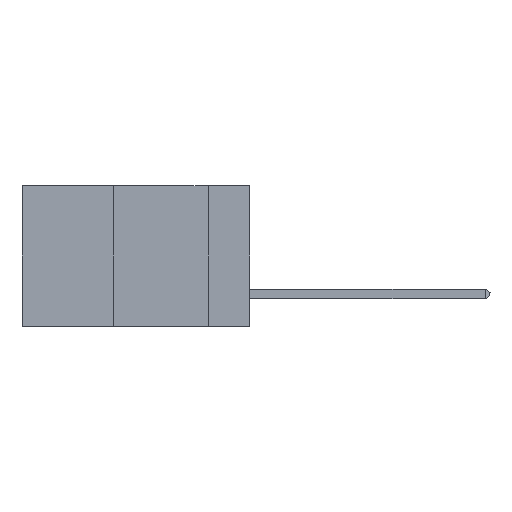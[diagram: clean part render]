
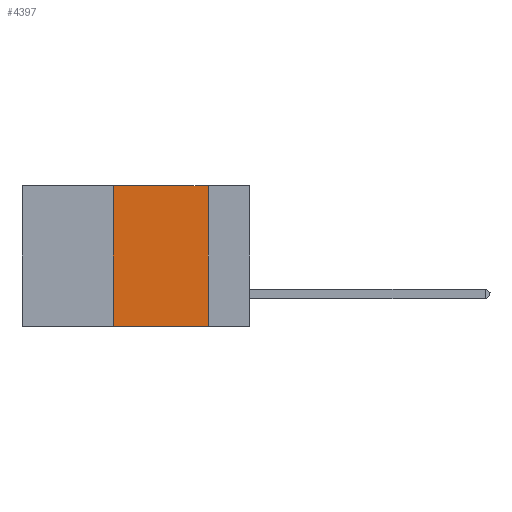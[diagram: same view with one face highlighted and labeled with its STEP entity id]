
A CAD part, left-side view. The second image highlights one B-rep face of the part: STEP entity #4397.
In plain terms, the highlighted planar face has unit normal (-1, 0, 0).
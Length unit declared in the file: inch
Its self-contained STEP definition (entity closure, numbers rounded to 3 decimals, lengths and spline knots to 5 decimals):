
#483 = DIRECTION ( 'NONE',  ( 0., -1., 0. ) ) ;
#1816 = FACE_OUTER_BOUND ( 'NONE', #12351, .T. ) ;
#2091 = ORIENTED_EDGE ( 'NONE', *, *, #14370, .T. ) ;
#2584 = DIRECTION ( 'NONE',  ( 0., 0., 1. ) ) ;
#3149 = DIRECTION ( 'NONE',  ( 0., 0., -1. ) ) ;
#3611 = CARTESIAN_POINT ( 'NONE',  ( 0., 0.36, -0.37 ) ) ;
#4104 = CARTESIAN_POINT ( 'NONE',  ( 0., 0.36, 0. ) ) ;
#4364 = CARTESIAN_POINT ( 'NONE',  ( 0., 0.6, 0. ) ) ;
#4397 = ADVANCED_FACE ( 'NONE', ( #1816 ), #8337, .F. ) ;
#5243 = ORIENTED_EDGE ( 'NONE', *, *, #6333, .F. ) ;
#6111 = VECTOR ( 'NONE', #2584, 39.37008 ) ;
#6153 = VECTOR ( 'NONE', #15186, 39.37008 ) ;
#6333 = EDGE_CURVE ( 'NONE', #7489, #11087, #11162, .T. ) ;
#6347 = EDGE_CURVE ( 'NONE', #11087, #14447, #15627, .T. ) ;
#6840 = AXIS2_PLACEMENT_3D ( 'NONE', #4364, #13334, #10800 ) ;
#7453 = CARTESIAN_POINT ( 'NONE',  ( 0., 0.11, 0. ) ) ;
#7489 = VERTEX_POINT ( 'NONE', #4104 ) ;
#8337 = PLANE ( 'NONE',  #6840 ) ;
#9461 = EDGE_CURVE ( 'NONE', #14302, #7489, #11856, .T. ) ;
#9681 = CARTESIAN_POINT ( 'NONE',  ( 0., 0.11, 0. ) ) ;
#10363 = VECTOR ( 'NONE', #483, 39.37008 ) ;
#10380 = CARTESIAN_POINT ( 'NONE',  ( 0., 0.36, 0. ) ) ;
#10589 = CARTESIAN_POINT ( 'NONE',  ( 0., 0.11, -0.37 ) ) ;
#10800 = DIRECTION ( 'NONE',  ( 0., 0., -1. ) ) ;
#10982 = CARTESIAN_POINT ( 'NONE',  ( 0., 0.6, 0. ) ) ;
#11087 = VERTEX_POINT ( 'NONE', #7453 ) ;
#11162 = LINE ( 'NONE', #10982, #10363 ) ;
#11588 = ORIENTED_EDGE ( 'NONE', *, *, #9461, .F. ) ;
#11856 = LINE ( 'NONE', #10380, #6111 ) ;
#11869 = ORIENTED_EDGE ( 'NONE', *, *, #6347, .F. ) ;
#12351 = EDGE_LOOP ( 'NONE', ( #11869, #5243, #11588, #2091 ) ) ;
#13334 = DIRECTION ( 'NONE',  ( 1., 0., 0. ) ) ;
#13348 = CARTESIAN_POINT ( 'NONE',  ( 0., 0.6, -0.37 ) ) ;
#14201 = VECTOR ( 'NONE', #3149, 39.37008 ) ;
#14302 = VERTEX_POINT ( 'NONE', #3611 ) ;
#14370 = EDGE_CURVE ( 'NONE', #14302, #14447, #16159, .T. ) ;
#14447 = VERTEX_POINT ( 'NONE', #10589 ) ;
#15186 = DIRECTION ( 'NONE',  ( 0., -1., 0. ) ) ;
#15627 = LINE ( 'NONE', #9681, #14201 ) ;
#16159 = LINE ( 'NONE', #13348, #6153 ) ;
